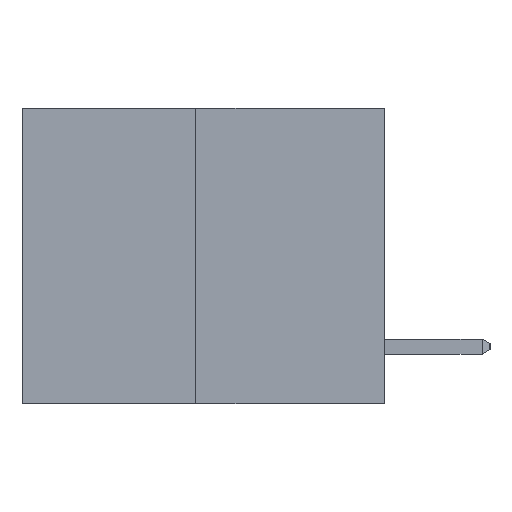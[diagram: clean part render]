
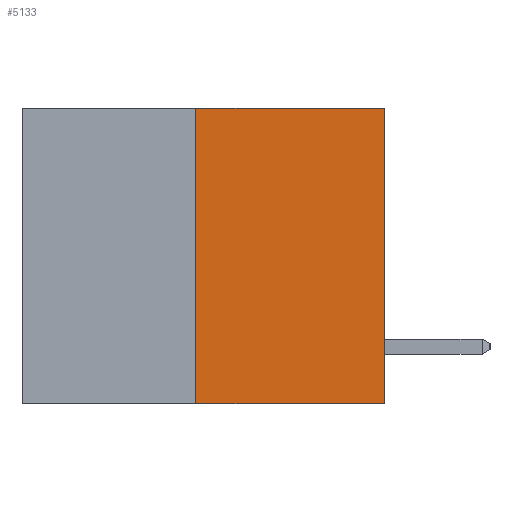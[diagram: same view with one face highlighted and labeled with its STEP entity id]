
A CAD part, left-side view. The second image highlights one B-rep face of the part: STEP entity #5133.
In plain terms, the highlighted planar face has unit normal (-1, 0, 0).
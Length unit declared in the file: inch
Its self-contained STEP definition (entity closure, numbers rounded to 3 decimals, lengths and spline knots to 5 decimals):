
#1331 = CARTESIAN_POINT ( 'NONE',  ( 0., 0., 0. ) ) ;
#1723 = CARTESIAN_POINT ( 'NONE',  ( 0., 0., 0. ) ) ;
#1782 = DIRECTION ( 'NONE',  ( 0., 0., 1. ) ) ;
#1981 = CARTESIAN_POINT ( 'NONE',  ( 0., 0., -0.49 ) ) ;
#2323 = DIRECTION ( 'NONE',  ( 0., -1., 0. ) ) ;
#2913 = VECTOR ( 'NONE', #16008, 39.37008 ) ;
#2928 = LINE ( 'NONE', #1723, #10435 ) ;
#3633 = CARTESIAN_POINT ( 'NONE',  ( 0., 0.312, 0. ) ) ;
#3674 = VERTEX_POINT ( 'NONE', #3633 ) ;
#4359 = EDGE_CURVE ( 'NONE', #4930, #3674, #8555, .T. ) ;
#4930 = VERTEX_POINT ( 'NONE', #9116 ) ;
#5083 = CARTESIAN_POINT ( 'NONE',  ( 0., 0.6, 0. ) ) ;
#5133 = ADVANCED_FACE ( 'NONE', ( #8102 ), #13099, .F. ) ;
#5534 = EDGE_CURVE ( 'NONE', #4930, #6500, #9383, .T. ) ;
#6500 = VERTEX_POINT ( 'NONE', #1981 ) ;
#6735 = CARTESIAN_POINT ( 'NONE',  ( 0., 0.6, -0.49 ) ) ;
#6895 = EDGE_CURVE ( 'NONE', #6500, #14140, #2928, .T. ) ;
#7017 = ORIENTED_EDGE ( 'NONE', *, *, #5534, .T. ) ;
#8102 = FACE_OUTER_BOUND ( 'NONE', #17163, .T. ) ;
#8198 = VECTOR ( 'NONE', #2323, 39.37008 ) ;
#8555 = LINE ( 'NONE', #14655, #8767 ) ;
#8767 = VECTOR ( 'NONE', #10774, 39.37008 ) ;
#8860 = DIRECTION ( 'NONE',  ( 1., 0., 0. ) ) ;
#9116 = CARTESIAN_POINT ( 'NONE',  ( 0., 0.312, -0.49 ) ) ;
#9383 = LINE ( 'NONE', #6735, #2913 ) ;
#10350 = ORIENTED_EDGE ( 'NONE', *, *, #11560, .F. ) ;
#10435 = VECTOR ( 'NONE', #1782, 39.37008 ) ;
#10771 = CARTESIAN_POINT ( 'NONE',  ( 0., 0.6, 0. ) ) ;
#10774 = DIRECTION ( 'NONE',  ( 0., 0., 1. ) ) ;
#10886 = AXIS2_PLACEMENT_3D ( 'NONE', #10771, #8860, #11285 ) ;
#11285 = DIRECTION ( 'NONE',  ( 0., 0., -1. ) ) ;
#11560 = EDGE_CURVE ( 'NONE', #3674, #14140, #12574, .T. ) ;
#12574 = LINE ( 'NONE', #5083, #8198 ) ;
#13099 = PLANE ( 'NONE',  #10886 ) ;
#14140 = VERTEX_POINT ( 'NONE', #1331 ) ;
#14332 = ORIENTED_EDGE ( 'NONE', *, *, #4359, .F. ) ;
#14655 = CARTESIAN_POINT ( 'NONE',  ( 0., 0.312, -0.49 ) ) ;
#16008 = DIRECTION ( 'NONE',  ( 0., -1., 0. ) ) ;
#16173 = ORIENTED_EDGE ( 'NONE', *, *, #6895, .T. ) ;
#17163 = EDGE_LOOP ( 'NONE', ( #14332, #7017, #16173, #10350 ) ) ;
